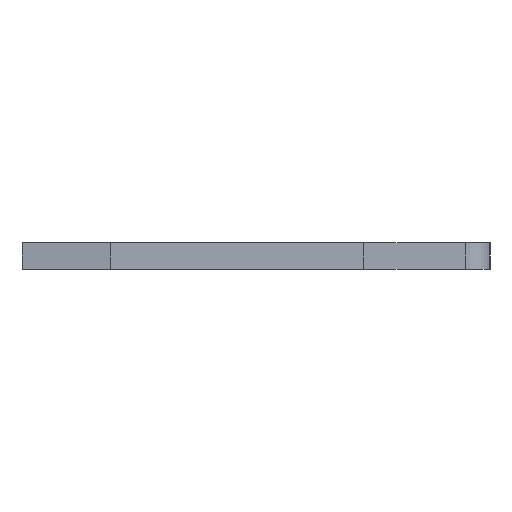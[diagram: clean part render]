
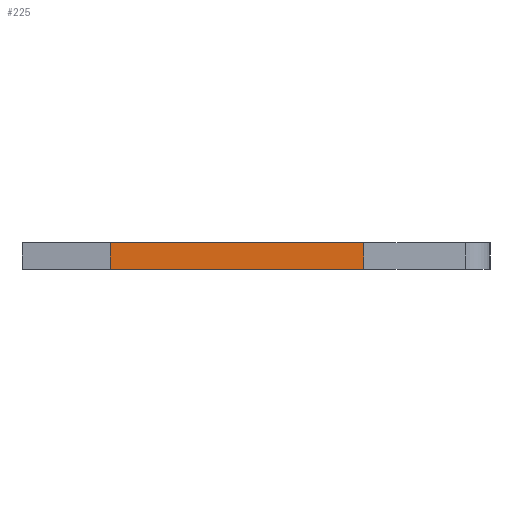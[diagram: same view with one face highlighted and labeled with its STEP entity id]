
A CAD part, left-side view. The second image highlights one B-rep face of the part: STEP entity #225.
In plain terms, the highlighted face is planar.
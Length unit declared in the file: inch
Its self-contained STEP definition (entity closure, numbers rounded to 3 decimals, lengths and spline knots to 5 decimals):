
#30 = VERTEX_POINT ( 'NONE', #1313 ) ;
#69 = VERTEX_POINT ( 'NONE', #1589 ) ;
#115 = ORIENTED_EDGE ( 'NONE', *, *, #1325, .T. ) ;
#123 = DIRECTION ( 'NONE',  ( 0., 1., 0. ) ) ;
#221 = ORIENTED_EDGE ( 'NONE', *, *, #256, .T. ) ;
#225 = ADVANCED_FACE ( 'NONE', ( #942 ), #1173, .F. ) ;
#256 = EDGE_CURVE ( 'NONE', #514, #30, #1742, .T. ) ;
#416 = CARTESIAN_POINT ( 'NONE',  ( 0.013, 0.146, -0.0575 ) ) ;
#514 = VERTEX_POINT ( 'NONE', #1781 ) ;
#594 = CARTESIAN_POINT ( 'NONE',  ( 0.013, 0.146, -0.0575 ) ) ;
#598 = LINE ( 'NONE', #1620, #682 ) ;
#601 = AXIS2_PLACEMENT_3D ( 'NONE', #594, #886, #1332 ) ;
#682 = VECTOR ( 'NONE', #123, 39.37008 ) ;
#703 = VECTOR ( 'NONE', #1491, 39.37008 ) ;
#712 = CARTESIAN_POINT ( 'NONE',  ( 0.013, 0.146, -0.0575 ) ) ;
#886 = DIRECTION ( 'NONE',  ( 0., 0., 1. ) ) ;
#893 = ORIENTED_EDGE ( 'NONE', *, *, #1365, .F. ) ;
#942 = FACE_OUTER_BOUND ( 'NONE', #1633, .T. ) ;
#1018 = LINE ( 'NONE', #416, #1857 ) ;
#1123 = VECTOR ( 'NONE', #1600, 39.37008 ) ;
#1146 = CARTESIAN_POINT ( 'NONE',  ( 0.013, -0.099, -0.0575 ) ) ;
#1173 = PLANE ( 'NONE',  #601 ) ;
#1233 = VERTEX_POINT ( 'NONE', #712 ) ;
#1245 = ORIENTED_EDGE ( 'NONE', *, *, #1506, .F. ) ;
#1263 = LINE ( 'NONE', #1146, #1123 ) ;
#1313 = CARTESIAN_POINT ( 'NONE',  ( -0.013, 0.146, -0.0575 ) ) ;
#1325 = EDGE_CURVE ( 'NONE', #69, #514, #1263, .T. ) ;
#1332 = DIRECTION ( 'NONE',  ( 1., 0., 0. ) ) ;
#1365 = EDGE_CURVE ( 'NONE', #69, #1233, #598, .T. ) ;
#1485 = CARTESIAN_POINT ( 'NONE',  ( -0.013, 0.146, -0.0575 ) ) ;
#1491 = DIRECTION ( 'NONE',  ( 0., 1., 0. ) ) ;
#1506 = EDGE_CURVE ( 'NONE', #1233, #30, #1018, .T. ) ;
#1589 = CARTESIAN_POINT ( 'NONE',  ( 0.013, -0.099, -0.0575 ) ) ;
#1600 = DIRECTION ( 'NONE',  ( -1., 0., 0. ) ) ;
#1620 = CARTESIAN_POINT ( 'NONE',  ( 0.013, 0.146, -0.0575 ) ) ;
#1633 = EDGE_LOOP ( 'NONE', ( #221, #1245, #893, #115 ) ) ;
#1742 = LINE ( 'NONE', #1485, #703 ) ;
#1751 = DIRECTION ( 'NONE',  ( -1., 0., 0. ) ) ;
#1781 = CARTESIAN_POINT ( 'NONE',  ( -0.013, -0.099, -0.0575 ) ) ;
#1857 = VECTOR ( 'NONE', #1751, 39.37008 ) ;
